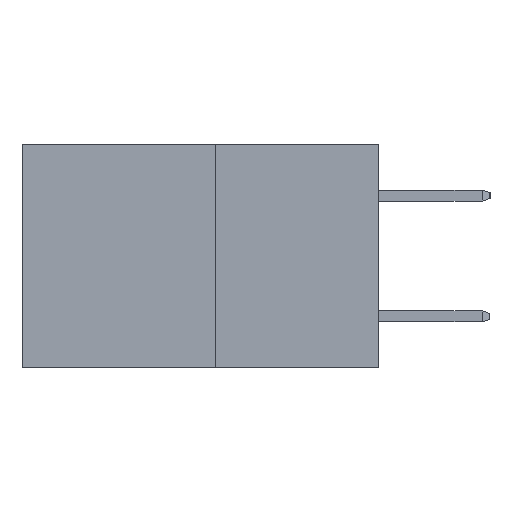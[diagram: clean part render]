
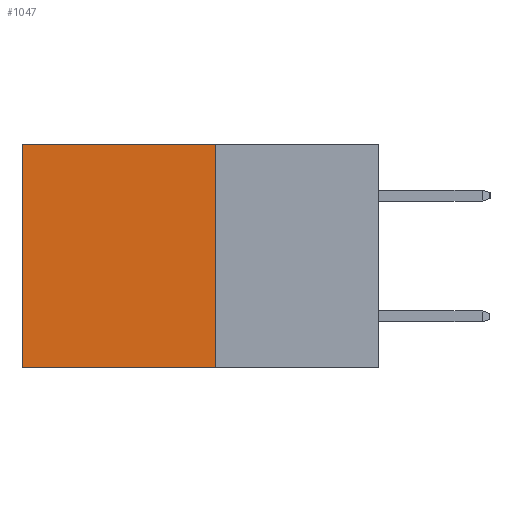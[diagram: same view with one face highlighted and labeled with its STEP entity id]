
A CAD part, left-side view. The second image highlights one B-rep face of the part: STEP entity #1047.
In plain terms, the highlighted planar face has unit normal (-1, 0, 0).
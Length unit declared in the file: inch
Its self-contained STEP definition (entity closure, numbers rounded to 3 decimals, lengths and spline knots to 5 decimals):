
#91 = AXIS2_PLACEMENT_3D ( 'NONE', #11640, #13519, #10987 ) ;
#110 = LINE ( 'NONE', #8488, #8577 ) ;
#777 = EDGE_CURVE ( 'NONE', #9233, #8343, #12126, .T. ) ;
#1047 = ADVANCED_FACE ( 'NONE', ( #11279 ), #11042, .F. ) ;
#1419 = CARTESIAN_POINT ( 'NONE',  ( 0.277, 0.27, -0.37 ) ) ;
#2428 = LINE ( 'NONE', #1419, #7901 ) ;
#3326 = ORIENTED_EDGE ( 'NONE', *, *, #7712, .F. ) ;
#3445 = ORIENTED_EDGE ( 'NONE', *, *, #4173, .F. ) ;
#4173 = EDGE_CURVE ( 'NONE', #4499, #7349, #8455, .T. ) ;
#4499 = VERTEX_POINT ( 'NONE', #4609 ) ;
#4609 = CARTESIAN_POINT ( 'NONE',  ( 0.277, 0.27, -0.37 ) ) ;
#6280 = CARTESIAN_POINT ( 'NONE',  ( 0.277, 0.59, 0. ) ) ;
#6456 = CARTESIAN_POINT ( 'NONE',  ( 0.277, 0.27, 0. ) ) ;
#6607 = DIRECTION ( 'NONE',  ( 0., 0., -1. ) ) ;
#7348 = ORIENTED_EDGE ( 'NONE', *, *, #9284, .T. ) ;
#7349 = VERTEX_POINT ( 'NONE', #8593 ) ;
#7712 = EDGE_CURVE ( 'NONE', #9233, #4499, #2428, .T. ) ;
#7901 = VECTOR ( 'NONE', #13666, 39.37008 ) ;
#8343 = VERTEX_POINT ( 'NONE', #6280 ) ;
#8455 = LINE ( 'NONE', #9325, #13846 ) ;
#8488 = CARTESIAN_POINT ( 'NONE',  ( 0.277, 0.59, -0.37 ) ) ;
#8577 = VECTOR ( 'NONE', #6607, 39.37008 ) ;
#8593 = CARTESIAN_POINT ( 'NONE',  ( 0.277, 0.59, -0.37 ) ) ;
#9233 = VERTEX_POINT ( 'NONE', #6456 ) ;
#9284 = EDGE_CURVE ( 'NONE', #8343, #7349, #110, .T. ) ;
#9325 = CARTESIAN_POINT ( 'NONE',  ( 0.277, 0.27, -0.37 ) ) ;
#9580 = VECTOR ( 'NONE', #11397, 39.37008 ) ;
#10020 = DIRECTION ( 'NONE',  ( 0., 1., 0. ) ) ;
#10032 = CARTESIAN_POINT ( 'NONE',  ( 0.277, 0.27, 0. ) ) ;
#10987 = DIRECTION ( 'NONE',  ( 0., 0., -1. ) ) ;
#11042 = PLANE ( 'NONE',  #91 ) ;
#11279 = FACE_OUTER_BOUND ( 'NONE', #12337, .T. ) ;
#11397 = DIRECTION ( 'NONE',  ( 0., 1., 0. ) ) ;
#11640 = CARTESIAN_POINT ( 'NONE',  ( 0.277, 0.27, -0.37 ) ) ;
#12126 = LINE ( 'NONE', #10032, #9580 ) ;
#12337 = EDGE_LOOP ( 'NONE', ( #7348, #3445, #3326, #14043 ) ) ;
#13519 = DIRECTION ( 'NONE',  ( 1., 0., 0. ) ) ;
#13666 = DIRECTION ( 'NONE',  ( 0., 0., -1. ) ) ;
#13846 = VECTOR ( 'NONE', #10020, 39.37008 ) ;
#14043 = ORIENTED_EDGE ( 'NONE', *, *, #777, .T. ) ;
